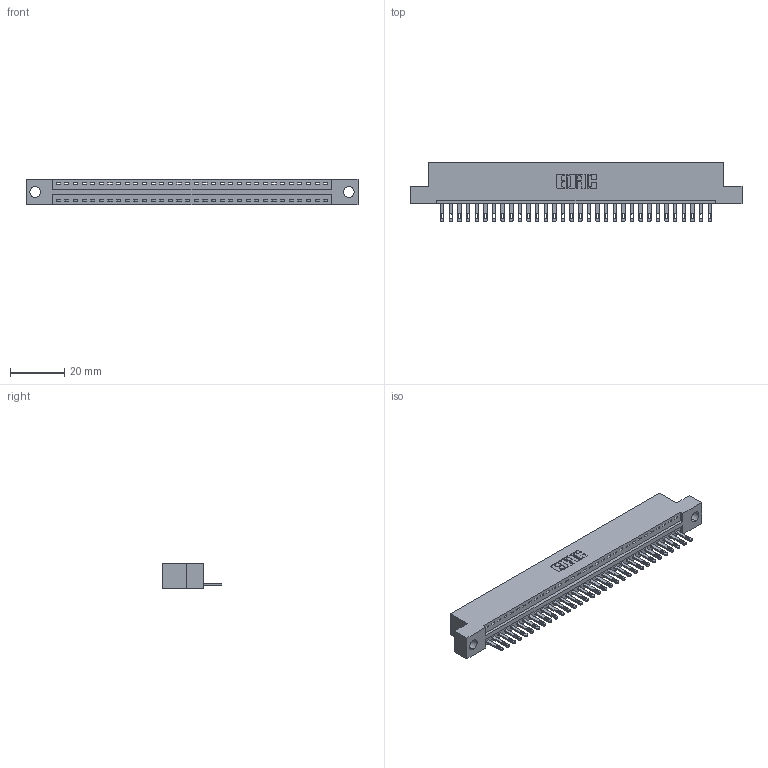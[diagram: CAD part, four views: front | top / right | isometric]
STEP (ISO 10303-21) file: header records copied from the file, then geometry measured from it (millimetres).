
FILE_DESCRIPTION (( 'STEP AP203' ), '1' );
FILE_NAME ('896-032-500-104.STEP', '2021-07-27T19:11:03', ( '' ), ( '' ), 'SwSTEP 2.0', 'SolidWorks 2020', '' );
FILE_SCHEMA (( 'CONFIG_CONTROL_DESIGN' ));
Length unit declared in the file: inch
Products named in the file (3): 846 Part_Flush Mounting Lugs - 0.156 Dia-TH; 345-292-001_345-293-100; 896-032-500-104
Assembly tree (33 placements, depth 2):
  896-032-500-104
    846 Part_Flush Mounting Lugs - 0.156 Dia-TH
    345-292-001_345-293-100  x32
Bounding box: 122.17 x 21.84 x 9.4 mm (x, y, z)
Volume: 11557.8 mm3; surface area: 14217.4 mm2
Topology: 33 solids, 33 shells, 1850 faces, 5705 edges, 3802 vertices
Faces by surface type: plane 1164, cylinder 686
Entity records: 21139 total; most frequent: CARTESIAN_POINT 3632, ORIENTED_EDGE 3598, DIRECTION 3219, EDGE_CURVE 1799, LINE 1535, VECTOR 1535, VERTEX_POINT 1198, AXIS2_PLACEMENT_3D 842
